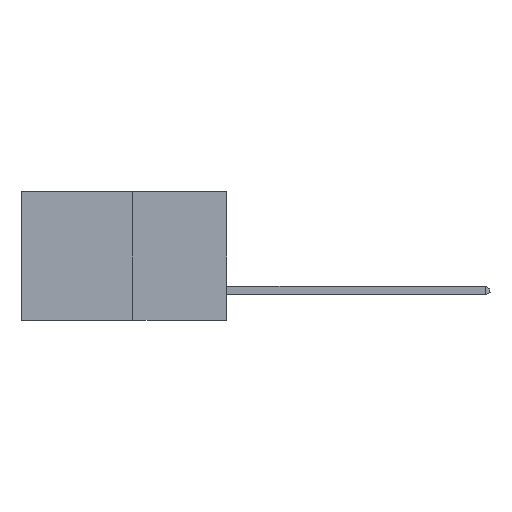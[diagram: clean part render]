
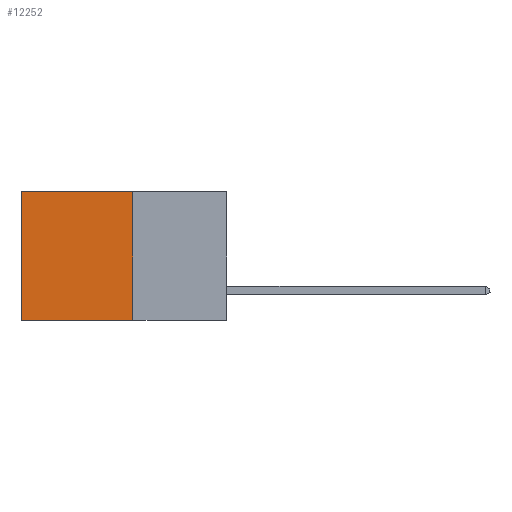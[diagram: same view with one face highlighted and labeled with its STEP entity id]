
A CAD part, left-side view. The second image highlights one B-rep face of the part: STEP entity #12252.
In plain terms, the highlighted planar face has unit normal (-1, 0, 0).
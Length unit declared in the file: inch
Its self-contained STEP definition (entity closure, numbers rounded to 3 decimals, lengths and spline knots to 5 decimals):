
#130 = EDGE_CURVE ( 'NONE', #17347, #11217, #14608, .T. ) ;
#158 = PLANE ( 'NONE',  #729 ) ;
#729 = AXIS2_PLACEMENT_3D ( 'NONE', #11807, #3081, #13257 ) ;
#1910 = VERTEX_POINT ( 'NONE', #15995 ) ;
#2353 = ORIENTED_EDGE ( 'NONE', *, *, #4270, .T. ) ;
#2409 = CARTESIAN_POINT ( 'NONE',  ( 0.277, 0.59, -0.37 ) ) ;
#2956 = LINE ( 'NONE', #3308, #17978 ) ;
#2982 = VECTOR ( 'NONE', #15557, 39.37008 ) ;
#3063 = CARTESIAN_POINT ( 'NONE',  ( 0.277, 0.59, 0. ) ) ;
#3081 = DIRECTION ( 'NONE',  ( 1., 0., 0. ) ) ;
#3308 = CARTESIAN_POINT ( 'NONE',  ( 0.277, 0.27, -0.37 ) ) ;
#4126 = CARTESIAN_POINT ( 'NONE',  ( 0.277, 0.27, -0.37 ) ) ;
#4270 = EDGE_CURVE ( 'NONE', #8021, #17347, #4835, .T. ) ;
#4275 = DIRECTION ( 'NONE',  ( 0., 1., 0. ) ) ;
#4391 = VECTOR ( 'NONE', #4275, 39.37008 ) ;
#4835 = LINE ( 'NONE', #10059, #4391 ) ;
#6049 = EDGE_CURVE ( 'NONE', #8021, #1910, #15464, .T. ) ;
#6816 = CARTESIAN_POINT ( 'NONE',  ( 0.277, 0.59, -0.37 ) ) ;
#7058 = DIRECTION ( 'NONE',  ( 0., 0., -1. ) ) ;
#8021 = VERTEX_POINT ( 'NONE', #13178 ) ;
#9084 = EDGE_CURVE ( 'NONE', #1910, #11217, #2956, .T. ) ;
#10059 = CARTESIAN_POINT ( 'NONE',  ( 0.277, 0.27, 0. ) ) ;
#11217 = VERTEX_POINT ( 'NONE', #6816 ) ;
#11807 = CARTESIAN_POINT ( 'NONE',  ( 0.277, 0.27, -0.37 ) ) ;
#12252 = ADVANCED_FACE ( 'NONE', ( #16338 ), #158, .F. ) ;
#12387 = EDGE_LOOP ( 'NONE', ( #18033, #18267, #13753, #2353 ) ) ;
#13178 = CARTESIAN_POINT ( 'NONE',  ( 0.277, 0.27, 0. ) ) ;
#13257 = DIRECTION ( 'NONE',  ( 0., 0., -1. ) ) ;
#13753 = ORIENTED_EDGE ( 'NONE', *, *, #6049, .F. ) ;
#14560 = VECTOR ( 'NONE', #7058, 39.37008 ) ;
#14608 = LINE ( 'NONE', #2409, #2982 ) ;
#15464 = LINE ( 'NONE', #4126, #14560 ) ;
#15557 = DIRECTION ( 'NONE',  ( 0., 0., -1. ) ) ;
#15995 = CARTESIAN_POINT ( 'NONE',  ( 0.277, 0.27, -0.37 ) ) ;
#16338 = FACE_OUTER_BOUND ( 'NONE', #12387, .T. ) ;
#16419 = DIRECTION ( 'NONE',  ( 0., 1., 0. ) ) ;
#17347 = VERTEX_POINT ( 'NONE', #3063 ) ;
#17978 = VECTOR ( 'NONE', #16419, 39.37008 ) ;
#18033 = ORIENTED_EDGE ( 'NONE', *, *, #130, .T. ) ;
#18267 = ORIENTED_EDGE ( 'NONE', *, *, #9084, .F. ) ;
